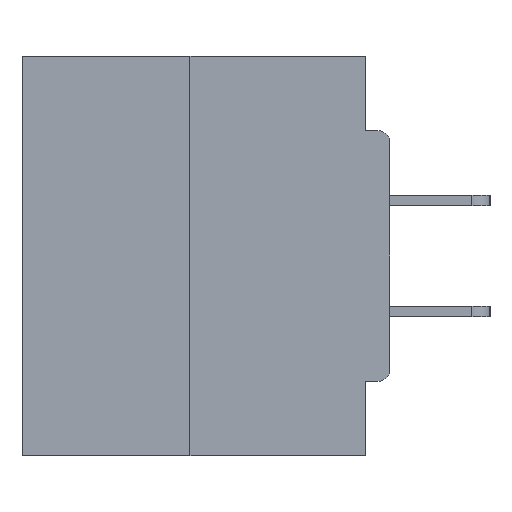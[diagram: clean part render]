
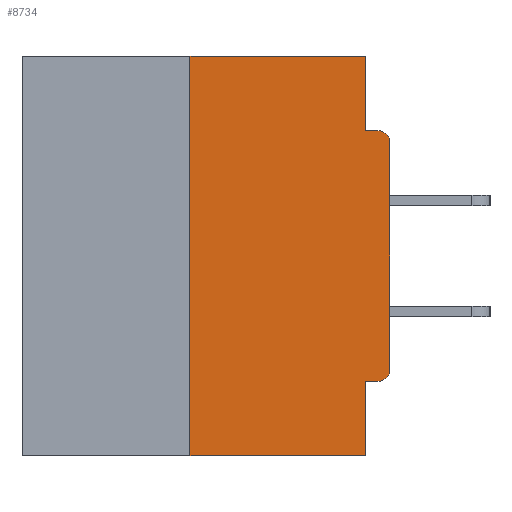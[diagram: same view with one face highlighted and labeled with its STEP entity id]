
A CAD part, left-side view. The second image highlights one B-rep face of the part: STEP entity #8734.
In plain terms, the highlighted planar face has unit normal (-1, 0, 0).
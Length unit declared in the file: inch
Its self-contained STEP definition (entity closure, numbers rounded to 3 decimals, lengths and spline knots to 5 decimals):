
#985 = ORIENTED_EDGE ( 'NONE', *, *, #13982, .F. ) ;
#1093 = VERTEX_POINT ( 'NONE', #7621 ) ;
#1437 = ORIENTED_EDGE ( 'NONE', *, *, #23507, .F. ) ;
#1728 = VERTEX_POINT ( 'NONE', #3754 ) ;
#1775 = EDGE_CURVE ( 'NONE', #13636, #11613, #23254, .T. ) ;
#1947 = CARTESIAN_POINT ( 'NONE',  ( 0., 0.031, 0. ) ) ;
#1993 = CARTESIAN_POINT ( 'NONE',  ( 0., 0., 0. ) ) ;
#2014 = ORIENTED_EDGE ( 'NONE', *, *, #8739, .T. ) ;
#2114 = VECTOR ( 'NONE', #28117, 39.37008 ) ;
#2317 = VECTOR ( 'NONE', #8958, 39.37008 ) ;
#2740 = CARTESIAN_POINT ( 'NONE',  ( 0., 0.46, 0. ) ) ;
#3019 = DIRECTION ( 'NONE',  ( -1., 0., 0. ) ) ;
#3459 = DIRECTION ( 'NONE',  ( 0., 0., -1. ) ) ;
#3611 = VECTOR ( 'NONE', #18644, 39.37008 ) ;
#3718 = ORIENTED_EDGE ( 'NONE', *, *, #12891, .T. ) ;
#3754 = CARTESIAN_POINT ( 'NONE',  ( 0., 0.031, -0.5 ) ) ;
#4678 = CIRCLE ( 'NONE', #27145, 0.015 ) ;
#5103 = ORIENTED_EDGE ( 'NONE', *, *, #32152, .T. ) ;
#5161 = VERTEX_POINT ( 'NONE', #18331 ) ;
#5423 = ORIENTED_EDGE ( 'NONE', *, *, #20848, .F. ) ;
#5701 = LINE ( 'NONE', #15688, #3611 ) ;
#6570 = ORIENTED_EDGE ( 'NONE', *, *, #16099, .F. ) ;
#6783 = LINE ( 'NONE', #31716, #17339 ) ;
#6928 = DIRECTION ( 'NONE',  ( -1., 0., 0. ) ) ;
#6987 = CARTESIAN_POINT ( 'NONE',  ( 0., 0.25, -0.5 ) ) ;
#7621 = CARTESIAN_POINT ( 'NONE',  ( 0., 0.015, -0.0935 ) ) ;
#7731 = CARTESIAN_POINT ( 'NONE',  ( 0., 0.015, -0.1085 ) ) ;
#8734 = ADVANCED_FACE ( 'NONE', ( #26390 ), #19483, .F. ) ;
#8739 = EDGE_CURVE ( 'NONE', #10496, #9885, #21484, .T. ) ;
#8958 = DIRECTION ( 'NONE',  ( 0., 0., -1. ) ) ;
#9022 = DIRECTION ( 'NONE',  ( 0., 0., -1. ) ) ;
#9223 = CARTESIAN_POINT ( 'NONE',  ( 0., 0.015, -0.3915 ) ) ;
#9885 = VERTEX_POINT ( 'NONE', #18947 ) ;
#10293 = CARTESIAN_POINT ( 'NONE',  ( 0., 0.46, -0.5 ) ) ;
#10496 = VERTEX_POINT ( 'NONE', #24614 ) ;
#11193 = VERTEX_POINT ( 'NONE', #6987 ) ;
#11467 = DIRECTION ( 'NONE',  ( 1., 0., 0. ) ) ;
#11553 = CIRCLE ( 'NONE', #20974, 0.015 ) ;
#11613 = VERTEX_POINT ( 'NONE', #22472 ) ;
#11675 = CARTESIAN_POINT ( 'NONE',  ( 0., 0.031, -0.4065 ) ) ;
#11741 = VECTOR ( 'NONE', #27003, 39.37008 ) ;
#12272 = EDGE_CURVE ( 'NONE', #11193, #28072, #5701, .T. ) ;
#12891 = EDGE_CURVE ( 'NONE', #9885, #1093, #4678, .T. ) ;
#12967 = DIRECTION ( 'NONE',  ( 0., 0., -1. ) ) ;
#13249 = CARTESIAN_POINT ( 'NONE',  ( 0., 0.031, -0.5 ) ) ;
#13636 = VERTEX_POINT ( 'NONE', #30775 ) ;
#13682 = VECTOR ( 'NONE', #27497, 39.37008 ) ;
#13982 = EDGE_CURVE ( 'NONE', #28072, #13636, #27769, .T. ) ;
#14769 = EDGE_CURVE ( 'NONE', #5161, #10496, #11553, .T. ) ;
#15688 = CARTESIAN_POINT ( 'NONE',  ( 0., 0.25, 0. ) ) ;
#16099 = EDGE_CURVE ( 'NONE', #21234, #1728, #21292, .T. ) ;
#17018 = LINE ( 'NONE', #22270, #11741 ) ;
#17339 = VECTOR ( 'NONE', #28472, 39.37008 ) ;
#18331 = CARTESIAN_POINT ( 'NONE',  ( 0., 0.015, -0.4065 ) ) ;
#18644 = DIRECTION ( 'NONE',  ( 0., 0., 1. ) ) ;
#18947 = CARTESIAN_POINT ( 'NONE',  ( 0., 0., -0.1085 ) ) ;
#19483 = PLANE ( 'NONE',  #32181 ) ;
#20848 = EDGE_CURVE ( 'NONE', #5161, #21234, #6783, .T. ) ;
#20974 = AXIS2_PLACEMENT_3D ( 'NONE', #9223, #6928, #27206 ) ;
#21234 = VERTEX_POINT ( 'NONE', #11675 ) ;
#21292 = LINE ( 'NONE', #13249, #26253 ) ;
#21484 = LINE ( 'NONE', #1993, #26935 ) ;
#21551 = ORIENTED_EDGE ( 'NONE', *, *, #12272, .F. ) ;
#22270 = CARTESIAN_POINT ( 'NONE',  ( 0., 0., -0.0935 ) ) ;
#22472 = CARTESIAN_POINT ( 'NONE',  ( 0., 0.031, -0.0935 ) ) ;
#22940 = ORIENTED_EDGE ( 'NONE', *, *, #1775, .F. ) ;
#23254 = LINE ( 'NONE', #1947, #2317 ) ;
#23507 = EDGE_CURVE ( 'NONE', #11613, #1093, #17018, .T. ) ;
#23956 = CARTESIAN_POINT ( 'NONE',  ( 0., 0.46, 0. ) ) ;
#24614 = CARTESIAN_POINT ( 'NONE',  ( 0., 0., -0.3915 ) ) ;
#26253 = VECTOR ( 'NONE', #3459, 39.37008 ) ;
#26390 = FACE_OUTER_BOUND ( 'NONE', #31672, .T. ) ;
#26864 = DIRECTION ( 'NONE',  ( 0., 0., 1. ) ) ;
#26935 = VECTOR ( 'NONE', #26864, 39.37008 ) ;
#27003 = DIRECTION ( 'NONE',  ( 0., -1., 0. ) ) ;
#27145 = AXIS2_PLACEMENT_3D ( 'NONE', #7731, #3019, #12967 ) ;
#27163 = LINE ( 'NONE', #10293, #13682 ) ;
#27206 = DIRECTION ( 'NONE',  ( 0., 0., -1. ) ) ;
#27497 = DIRECTION ( 'NONE',  ( 0., -1., 0. ) ) ;
#27769 = LINE ( 'NONE', #2740, #2114 ) ;
#28072 = VERTEX_POINT ( 'NONE', #29404 ) ;
#28117 = DIRECTION ( 'NONE',  ( 0., -1., 0. ) ) ;
#28472 = DIRECTION ( 'NONE',  ( 0., 1., 0. ) ) ;
#29404 = CARTESIAN_POINT ( 'NONE',  ( 0., 0.25, 0. ) ) ;
#30775 = CARTESIAN_POINT ( 'NONE',  ( 0., 0.031, 0. ) ) ;
#31207 = ORIENTED_EDGE ( 'NONE', *, *, #14769, .T. ) ;
#31672 = EDGE_LOOP ( 'NONE', ( #985, #21551, #5103, #6570, #5423, #31207, #2014, #3718, #1437, #22940 ) ) ;
#31716 = CARTESIAN_POINT ( 'NONE',  ( 0., 0., -0.4065 ) ) ;
#32152 = EDGE_CURVE ( 'NONE', #11193, #1728, #27163, .T. ) ;
#32181 = AXIS2_PLACEMENT_3D ( 'NONE', #23956, #11467, #9022 ) ;
